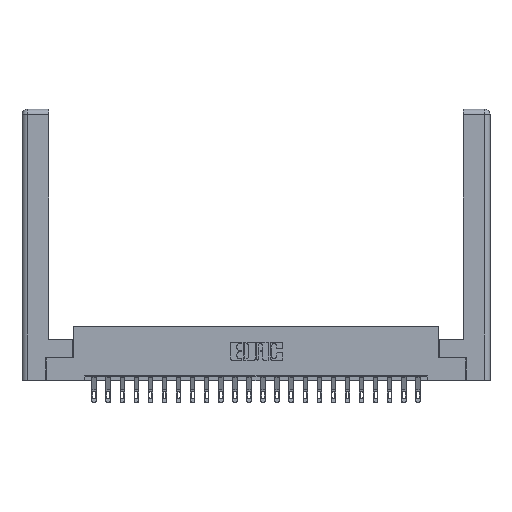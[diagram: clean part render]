
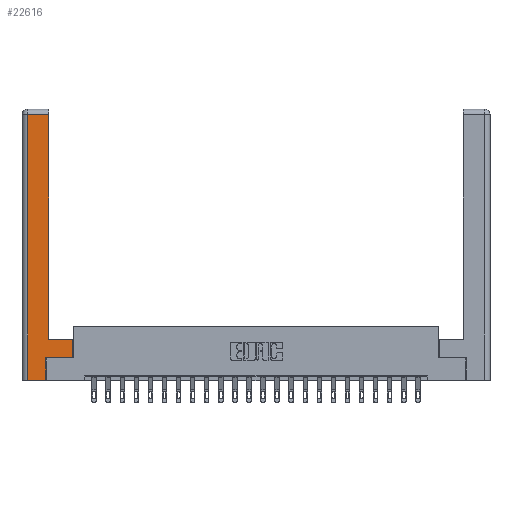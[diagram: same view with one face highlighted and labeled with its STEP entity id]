
A CAD part, top view. The second image highlights one B-rep face of the part: STEP entity #22616.
In plain terms, the highlighted planar face has unit normal (0, 0, 1).
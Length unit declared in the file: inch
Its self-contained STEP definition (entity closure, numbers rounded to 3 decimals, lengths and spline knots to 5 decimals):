
#409 = ORIENTED_EDGE ( 'NONE', *, *, #19966, .T. ) ;
#970 = CARTESIAN_POINT ( 'NONE',  ( 0.265, 0.245, 0. ) ) ;
#1142 = EDGE_CURVE ( 'NONE', #6751, #22484, #9428, .T. ) ;
#1383 = CARTESIAN_POINT ( 'NONE',  ( 0.265, 0., 0. ) ) ;
#1761 = AXIS2_PLACEMENT_3D ( 'NONE', #21412, #23282, #8328 ) ;
#2020 = ORIENTED_EDGE ( 'NONE', *, *, #5210, .T. ) ;
#2157 = VECTOR ( 'NONE', #19951, 39.37008 ) ;
#2160 = LINE ( 'NONE', #1383, #11441 ) ;
#2333 = EDGE_CURVE ( 'NONE', #22599, #12621, #8466, .T. ) ;
#2788 = CARTESIAN_POINT ( 'NONE',  ( 0.565, 0.45, 0. ) ) ;
#3045 = DIRECTION ( 'NONE',  ( -1., 0., 0. ) ) ;
#4263 = DIRECTION ( 'NONE',  ( 0., 1., 0. ) ) ;
#4481 = DIRECTION ( 'NONE',  ( 0., 1., 0. ) ) ;
#4595 = EDGE_CURVE ( 'NONE', #9648, #8726, #2160, .T. ) ;
#4902 = CARTESIAN_POINT ( 'NONE',  ( 0.265, 0., 0. ) ) ;
#5136 = DIRECTION ( 'NONE',  ( 1., 0., 0. ) ) ;
#5210 = EDGE_CURVE ( 'NONE', #12621, #17359, #17389, .T. ) ;
#5523 = CARTESIAN_POINT ( 'NONE',  ( 0.565, 0.245, 0. ) ) ;
#6116 = CARTESIAN_POINT ( 'NONE',  ( 0.295, 3., 0. ) ) ;
#6642 = EDGE_CURVE ( 'NONE', #16086, #9648, #16735, .T. ) ;
#6751 = VERTEX_POINT ( 'NONE', #9350 ) ;
#7262 = CARTESIAN_POINT ( 'NONE',  ( 0.0615, 0., 0. ) ) ;
#7590 = LINE ( 'NONE', #970, #23121 ) ;
#7936 = CARTESIAN_POINT ( 'NONE',  ( 0.565, 0.45, 0. ) ) ;
#8328 = DIRECTION ( 'NONE',  ( -1., 0., 0. ) ) ;
#8466 = LINE ( 'NONE', #11591, #16214 ) ;
#8726 = VERTEX_POINT ( 'NONE', #4902 ) ;
#9350 = CARTESIAN_POINT ( 'NONE',  ( 0.265, 0.245, 0. ) ) ;
#9428 = LINE ( 'NONE', #5523, #2157 ) ;
#9648 = VERTEX_POINT ( 'NONE', #7262 ) ;
#10367 = FACE_OUTER_BOUND ( 'NONE', #11062, .T. ) ;
#10450 = LINE ( 'NONE', #19590, #11630 ) ;
#11062 = EDGE_LOOP ( 'NONE', ( #2020, #409, #22199, #15677, #16069, #17272, #14794, #21844 ) ) ;
#11441 = VECTOR ( 'NONE', #5136, 39.37008 ) ;
#11591 = CARTESIAN_POINT ( 'NONE',  ( 0.295, 0.45, 0. ) ) ;
#11630 = VECTOR ( 'NONE', #3045, 39.37008 ) ;
#11660 = CARTESIAN_POINT ( 'NONE',  ( 0.565, 0.245, 0. ) ) ;
#12621 = VERTEX_POINT ( 'NONE', #13115 ) ;
#13115 = CARTESIAN_POINT ( 'NONE',  ( 0.295, 0.45, 0. ) ) ;
#14794 = ORIENTED_EDGE ( 'NONE', *, *, #16553, .T. ) ;
#15081 = VECTOR ( 'NONE', #21715, 39.37008 ) ;
#15315 = EDGE_CURVE ( 'NONE', #8726, #6751, #7590, .T. ) ;
#15677 = ORIENTED_EDGE ( 'NONE', *, *, #4595, .T. ) ;
#16069 = ORIENTED_EDGE ( 'NONE', *, *, #15315, .T. ) ;
#16086 = VERTEX_POINT ( 'NONE', #21680 ) ;
#16214 = VECTOR ( 'NONE', #16861, 39.37008 ) ;
#16553 = EDGE_CURVE ( 'NONE', #22484, #22599, #18936, .T. ) ;
#16735 = LINE ( 'NONE', #18167, #15081 ) ;
#16861 = DIRECTION ( 'NONE',  ( -1., 0., 0. ) ) ;
#17272 = ORIENTED_EDGE ( 'NONE', *, *, #1142, .T. ) ;
#17359 = VERTEX_POINT ( 'NONE', #19622 ) ;
#17389 = LINE ( 'NONE', #6116, #20561 ) ;
#18167 = CARTESIAN_POINT ( 'NONE',  ( 0.0615, 0., 0. ) ) ;
#18936 = LINE ( 'NONE', #7936, #20093 ) ;
#19576 = PLANE ( 'NONE',  #1761 ) ;
#19590 = CARTESIAN_POINT ( 'NONE',  ( 0.0615, 2.94, 0. ) ) ;
#19622 = CARTESIAN_POINT ( 'NONE',  ( 0.295, 2.94, 0. ) ) ;
#19951 = DIRECTION ( 'NONE',  ( 1., 0., 0. ) ) ;
#19966 = EDGE_CURVE ( 'NONE', #17359, #16086, #10450, .T. ) ;
#20093 = VECTOR ( 'NONE', #4263, 39.37008 ) ;
#20561 = VECTOR ( 'NONE', #4481, 39.37008 ) ;
#21071 = DIRECTION ( 'NONE',  ( 0., 1., 0. ) ) ;
#21412 = CARTESIAN_POINT ( 'NONE',  ( 0., 0., 0. ) ) ;
#21680 = CARTESIAN_POINT ( 'NONE',  ( 0.0615, 2.94, 0. ) ) ;
#21715 = DIRECTION ( 'NONE',  ( 0., -1., 0. ) ) ;
#21844 = ORIENTED_EDGE ( 'NONE', *, *, #2333, .T. ) ;
#22199 = ORIENTED_EDGE ( 'NONE', *, *, #6642, .T. ) ;
#22484 = VERTEX_POINT ( 'NONE', #11660 ) ;
#22599 = VERTEX_POINT ( 'NONE', #2788 ) ;
#22616 = ADVANCED_FACE ( 'NONE', ( #10367 ), #19576, .F. ) ;
#23121 = VECTOR ( 'NONE', #21071, 39.37008 ) ;
#23282 = DIRECTION ( 'NONE',  ( 0., 0., -1. ) ) ;
